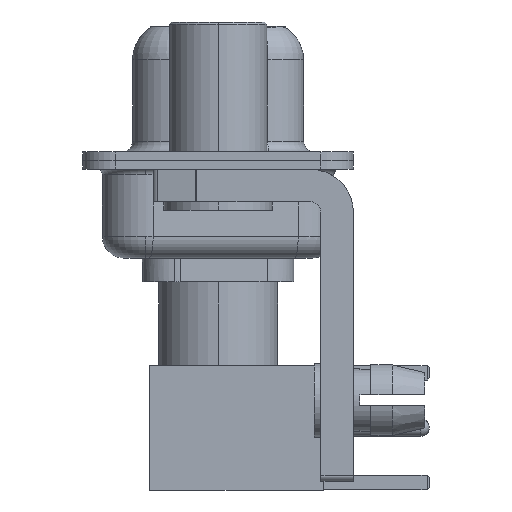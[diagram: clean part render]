
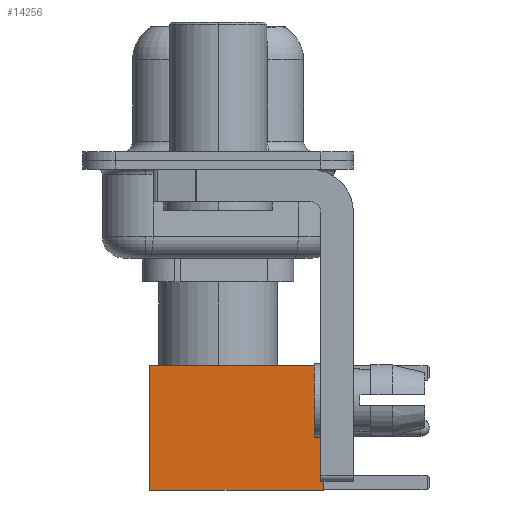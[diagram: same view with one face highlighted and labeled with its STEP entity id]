
A CAD part, left-side view. The second image highlights one B-rep face of the part: STEP entity #14256.
In plain terms, the highlighted face is planar.
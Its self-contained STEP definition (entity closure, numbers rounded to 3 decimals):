
#59 = CARTESIAN_POINT ( 'NONE',  ( 2.875, 2.875, 0. ) ) ;
#1982 = VECTOR ( 'NONE', #5205, 1000. ) ;
#2222 = CARTESIAN_POINT ( 'NONE',  ( 0., 2.875, 8. ) ) ;
#2289 = VECTOR ( 'NONE', #10301, 1000. ) ;
#3178 = FACE_OUTER_BOUND ( 'NONE', #4814, .T. ) ;
#3387 = EDGE_CURVE ( 'NONE', #3467, #11119, #13642, .T. ) ;
#3467 = VERTEX_POINT ( 'NONE', #8419 ) ;
#3532 = CARTESIAN_POINT ( 'NONE',  ( 0., 2.875, 0. ) ) ;
#3574 = ORIENTED_EDGE ( 'NONE', *, *, #3387, .T. ) ;
#4814 = EDGE_LOOP ( 'NONE', ( #8220, #3574, #7760, #15327 ) ) ;
#5086 = LINE ( 'NONE', #8442, #1982 ) ;
#5205 = DIRECTION ( 'NONE',  ( 0., 0., -1. ) ) ;
#7760 = ORIENTED_EDGE ( 'NONE', *, *, #15001, .F. ) ;
#8220 = ORIENTED_EDGE ( 'NONE', *, *, #20765, .T. ) ;
#8350 = CARTESIAN_POINT ( 'NONE',  ( 2.875, 2.875, 8. ) ) ;
#8419 = CARTESIAN_POINT ( 'NONE',  ( 2.875, 2.875, 0. ) ) ;
#8442 = CARTESIAN_POINT ( 'NONE',  ( 2.875, 2.875, 0. ) ) ;
#9444 = VECTOR ( 'NONE', #16117, 1000. ) ;
#9507 = AXIS2_PLACEMENT_3D ( 'NONE', #59, #12160, #13621 ) ;
#9978 = DIRECTION ( 'NONE',  ( 0., 0., -1. ) ) ;
#10301 = DIRECTION ( 'NONE',  ( -1., 0., 0. ) ) ;
#11119 = VERTEX_POINT ( 'NONE', #15982 ) ;
#12160 = DIRECTION ( 'NONE',  ( 0., 1., 0. ) ) ;
#12289 = CARTESIAN_POINT ( 'NONE',  ( -2.875, 2.875, 8. ) ) ;
#12659 = LINE ( 'NONE', #2222, #9444 ) ;
#13104 = CARTESIAN_POINT ( 'NONE',  ( -2.875, 2.875, 0. ) ) ;
#13621 = DIRECTION ( 'NONE',  ( 0., 0., 1. ) ) ;
#13642 = LINE ( 'NONE', #3532, #2289 ) ;
#14256 = ADVANCED_FACE ( 'NONE', ( #3178 ), #18541, .T. ) ;
#15001 = EDGE_CURVE ( 'NONE', #20084, #11119, #15007, .T. ) ;
#15007 = LINE ( 'NONE', #13104, #15940 ) ;
#15327 = ORIENTED_EDGE ( 'NONE', *, *, #20958, .F. ) ;
#15940 = VECTOR ( 'NONE', #9978, 1000. ) ;
#15982 = CARTESIAN_POINT ( 'NONE',  ( -2.875, 2.875, 0. ) ) ;
#16117 = DIRECTION ( 'NONE',  ( -1., 0., 0. ) ) ;
#18541 = PLANE ( 'NONE',  #9507 ) ;
#18891 = VERTEX_POINT ( 'NONE', #8350 ) ;
#20084 = VERTEX_POINT ( 'NONE', #12289 ) ;
#20765 = EDGE_CURVE ( 'NONE', #18891, #3467, #5086, .T. ) ;
#20958 = EDGE_CURVE ( 'NONE', #18891, #20084, #12659, .T. ) ;
